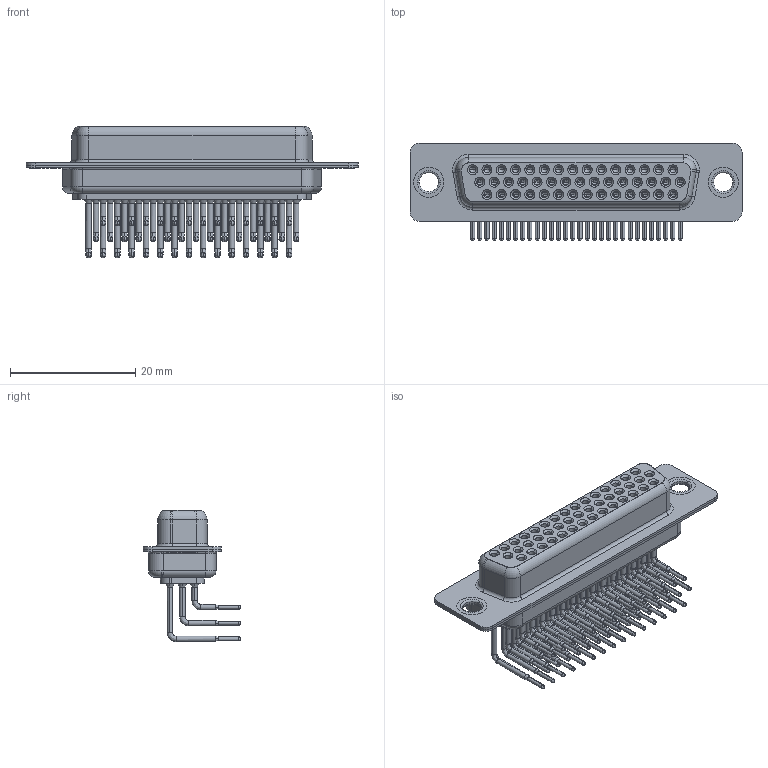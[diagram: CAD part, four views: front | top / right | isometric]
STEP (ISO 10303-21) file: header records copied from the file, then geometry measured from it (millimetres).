
FILE_DESCRIPTION (( 'STEP AP203' ), '1' );
FILE_NAME ('634-M44-663-BT1.STEP', '2018-09-28T01:45:25', ( '' ), ( '' ), 'SwSTEP 2.0', 'SolidWorks 2016', '' );
FILE_SCHEMA (( 'CONFIG_CONTROL_DESIGN' ));
Length unit declared in the file: millimetre
Products named in the file (8): 634-M44-663-BT1; 634M Housing_44 Contacts; 634M Shell Front_44 Contacts; 634M Shell Rear_44 Contacts; 634M Contact Row 1; 634M Contact Row 2; 634M Contact Row 3; 634M Thru Hole Rivet
Assembly tree (49 placements, depth 2):
  634-M44-663-BT1
    634M Housing_44 Contacts
    634M Shell Front_44 Contacts
    634M Shell Rear_44 Contacts
    634M Contact Row 1  x15
    634M Contact Row 2  x15
    634M Contact Row 3  x14
    634M Thru Hole Rivet  x2
Bounding box: 53.05 x 15.6 x 21.02 mm (x, y, z)
Volume: 3758.3 mm3; surface area: 12887.8 mm2
Topology: 49 solids, 49 shells, 2585 faces, 6543 edges, 4111 vertices
Faces by surface type: cylinder 1133, plane 727, cone 484, bspline 176, torus 65
Entity records: 29016 total; most frequent: DIRECTION 5199, CARTESIAN_POINT 4857, ORIENTED_EDGE 4208, AXIS2_PLACEMENT_3D 2199, EDGE_CURVE 2104, VERTEX_POINT 1340, CIRCLE 1234, EDGE_LOOP 1174
